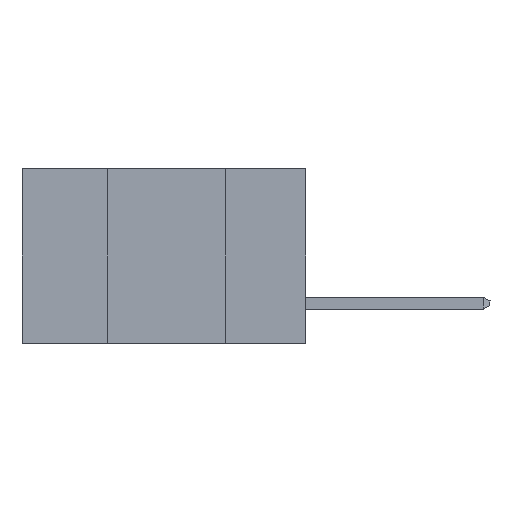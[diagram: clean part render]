
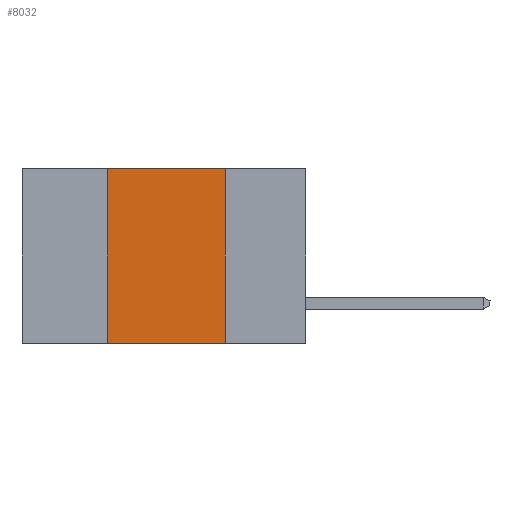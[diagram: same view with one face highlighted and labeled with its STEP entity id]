
A CAD part, left-side view. The second image highlights one B-rep face of the part: STEP entity #8032.
In plain terms, the highlighted planar face has unit normal (-1, 0, 0).
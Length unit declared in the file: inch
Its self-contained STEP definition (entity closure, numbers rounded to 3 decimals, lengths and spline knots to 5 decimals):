
#553 = CARTESIAN_POINT ( 'NONE',  ( 0., 0.17, 0. ) ) ;
#1791 = PLANE ( 'NONE',  #18427 ) ;
#2041 = ORIENTED_EDGE ( 'NONE', *, *, #11027, .F. ) ;
#2093 = DIRECTION ( 'NONE',  ( 0., 0., -1. ) ) ;
#3831 = DIRECTION ( 'NONE',  ( 0., 0., -1. ) ) ;
#5234 = VECTOR ( 'NONE', #16671, 39.37008 ) ;
#5636 = EDGE_CURVE ( 'NONE', #19348, #17793, #18136, .T. ) ;
#8032 = ADVANCED_FACE ( 'NONE', ( #12316 ), #1791, .F. ) ;
#8229 = VERTEX_POINT ( 'NONE', #22259 ) ;
#8279 = CARTESIAN_POINT ( 'NONE',  ( 0., 0.6, -0.37 ) ) ;
#8550 = CARTESIAN_POINT ( 'NONE',  ( 0., 0.17, 0. ) ) ;
#8599 = DIRECTION ( 'NONE',  ( 0., -1., 0. ) ) ;
#10852 = CARTESIAN_POINT ( 'NONE',  ( 0., 0.6, 0. ) ) ;
#11027 = EDGE_CURVE ( 'NONE', #17793, #17892, #13498, .T. ) ;
#12316 = FACE_OUTER_BOUND ( 'NONE', #27738, .T. ) ;
#12317 = VECTOR ( 'NONE', #15269, 39.37008 ) ;
#13498 = LINE ( 'NONE', #10852, #21365 ) ;
#13500 = ORIENTED_EDGE ( 'NONE', *, *, #5636, .F. ) ;
#15269 = DIRECTION ( 'NONE',  ( 0., 0., 1. ) ) ;
#16012 = VECTOR ( 'NONE', #2093, 39.37008 ) ;
#16671 = DIRECTION ( 'NONE',  ( 0., -1., 0. ) ) ;
#16890 = ORIENTED_EDGE ( 'NONE', *, *, #21678, .T. ) ;
#17793 = VERTEX_POINT ( 'NONE', #21390 ) ;
#17892 = VERTEX_POINT ( 'NONE', #553 ) ;
#18136 = LINE ( 'NONE', #20048, #12317 ) ;
#18427 = AXIS2_PLACEMENT_3D ( 'NONE', #27905, #25924, #3831 ) ;
#19348 = VERTEX_POINT ( 'NONE', #21064 ) ;
#19587 = LINE ( 'NONE', #8279, #5234 ) ;
#20048 = CARTESIAN_POINT ( 'NONE',  ( 0., 0.42, 0. ) ) ;
#20719 = ORIENTED_EDGE ( 'NONE', *, *, #24070, .F. ) ;
#21064 = CARTESIAN_POINT ( 'NONE',  ( 0., 0.42, -0.37 ) ) ;
#21365 = VECTOR ( 'NONE', #8599, 39.37008 ) ;
#21390 = CARTESIAN_POINT ( 'NONE',  ( 0., 0.42, 0. ) ) ;
#21678 = EDGE_CURVE ( 'NONE', #19348, #8229, #19587, .T. ) ;
#22259 = CARTESIAN_POINT ( 'NONE',  ( 0., 0.17, -0.37 ) ) ;
#24070 = EDGE_CURVE ( 'NONE', #17892, #8229, #24569, .T. ) ;
#24569 = LINE ( 'NONE', #8550, #16012 ) ;
#25924 = DIRECTION ( 'NONE',  ( 1., 0., 0. ) ) ;
#27738 = EDGE_LOOP ( 'NONE', ( #20719, #2041, #13500, #16890 ) ) ;
#27905 = CARTESIAN_POINT ( 'NONE',  ( 0., 0.6, 0. ) ) ;
